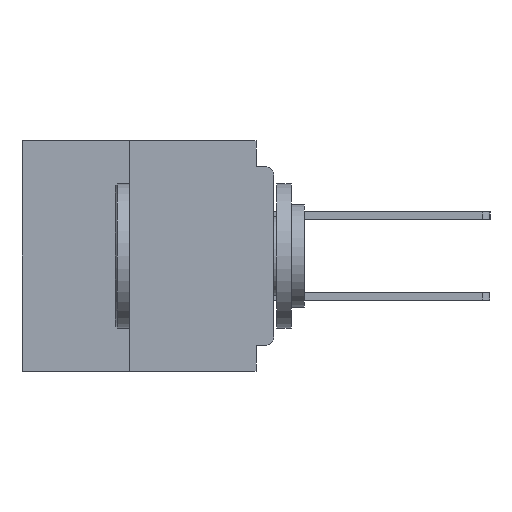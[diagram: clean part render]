
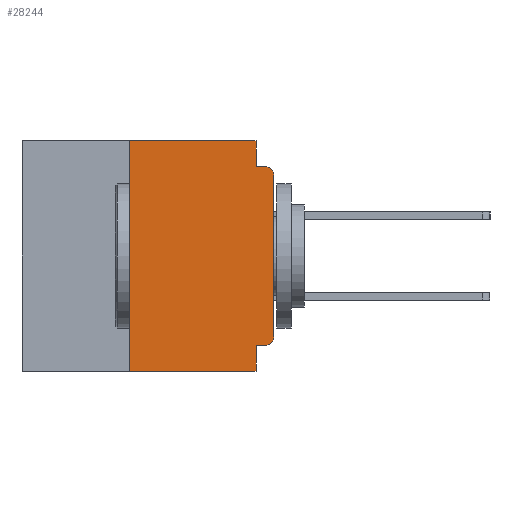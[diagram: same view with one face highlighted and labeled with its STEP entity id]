
A CAD part, left-side view. The second image highlights one B-rep face of the part: STEP entity #28244.
In plain terms, the highlighted planar face has unit normal (-1, 0, 0).
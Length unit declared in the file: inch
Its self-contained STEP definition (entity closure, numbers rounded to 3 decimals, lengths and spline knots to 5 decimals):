
#3299 = VERTEX_POINT ( 'NONE', #6352 ) ;
#4492 = VERTEX_POINT ( 'NONE', #36273 ) ;
#4686 = LINE ( 'NONE', #56543, #41906 ) ;
#5958 = ORIENTED_EDGE ( 'NONE', *, *, #50875, .F. ) ;
#6352 = CARTESIAN_POINT ( 'NONE',  ( 0., 0.25, -0.4 ) ) ;
#6396 = VECTOR ( 'NONE', #30634, 39.37008 ) ;
#6397 = CARTESIAN_POINT ( 'NONE',  ( 0., 0.437, -0.4 ) ) ;
#6936 = VERTEX_POINT ( 'NONE', #59837 ) ;
#7879 = CARTESIAN_POINT ( 'NONE',  ( 0., 0.031, 0. ) ) ;
#8286 = CIRCLE ( 'NONE', #15188, 0.015 ) ;
#8714 = VECTOR ( 'NONE', #12414, 39.37008 ) ;
#9457 = VECTOR ( 'NONE', #51533, 39.37008 ) ;
#12106 = CARTESIAN_POINT ( 'NONE',  ( 0., 0.015, -0.06 ) ) ;
#12159 = CARTESIAN_POINT ( 'NONE',  ( 0., 0.031, -0.355 ) ) ;
#12284 = CARTESIAN_POINT ( 'NONE',  ( 0., 0., -0.06 ) ) ;
#12414 = DIRECTION ( 'NONE',  ( 0., 0., 1. ) ) ;
#13117 = CARTESIAN_POINT ( 'NONE',  ( 0., 0.437, 0. ) ) ;
#14204 = CARTESIAN_POINT ( 'NONE',  ( 0., 0.015, -0.34 ) ) ;
#14446 = LINE ( 'NONE', #50013, #53010 ) ;
#15188 = AXIS2_PLACEMENT_3D ( 'NONE', #12106, #45990, #17058 ) ;
#16441 = VERTEX_POINT ( 'NONE', #31870 ) ;
#16653 = VECTOR ( 'NONE', #46979, 39.37008 ) ;
#17058 = DIRECTION ( 'NONE',  ( 0., 0., -1. ) ) ;
#17889 = ORIENTED_EDGE ( 'NONE', *, *, #33131, .T. ) ;
#19119 = DIRECTION ( 'NONE',  ( 0., 0., -1. ) ) ;
#19390 = PLANE ( 'NONE',  #32075 ) ;
#22426 = LINE ( 'NONE', #7879, #9457 ) ;
#22611 = DIRECTION ( 'NONE',  ( 0., 1., 0. ) ) ;
#22678 = VERTEX_POINT ( 'NONE', #55974 ) ;
#22692 = VERTEX_POINT ( 'NONE', #27287 ) ;
#23366 = ORIENTED_EDGE ( 'NONE', *, *, #61705, .F. ) ;
#24251 = DIRECTION ( 'NONE',  ( 1., 0., 0. ) ) ;
#24573 = LINE ( 'NONE', #46707, #35919 ) ;
#24841 = LINE ( 'NONE', #54201, #49025 ) ;
#25578 = EDGE_CURVE ( 'NONE', #45578, #22692, #14446, .T. ) ;
#25692 = EDGE_CURVE ( 'NONE', #55652, #22692, #8286, .T. ) ;
#25916 = DIRECTION ( 'NONE',  ( 0., -1., 0. ) ) ;
#26908 = VERTEX_POINT ( 'NONE', #12159 ) ;
#27287 = CARTESIAN_POINT ( 'NONE',  ( 0., 0.015, -0.045 ) ) ;
#28244 = ADVANCED_FACE ( 'NONE', ( #46644 ), #19390, .F. ) ;
#29496 = LINE ( 'NONE', #13117, #16653 ) ;
#30634 = DIRECTION ( 'NONE',  ( 0., -1., 0. ) ) ;
#30737 = LINE ( 'NONE', #6397, #6396 ) ;
#31812 = ORIENTED_EDGE ( 'NONE', *, *, #25692, .T. ) ;
#31870 = CARTESIAN_POINT ( 'NONE',  ( 0., 0.015, -0.355 ) ) ;
#32075 = AXIS2_PLACEMENT_3D ( 'NONE', #48321, #24251, #57952 ) ;
#32225 = EDGE_CURVE ( 'NONE', #4492, #45578, #22426, .T. ) ;
#32539 = DIRECTION ( 'NONE',  ( 0., 0., 1. ) ) ;
#33131 = EDGE_CURVE ( 'NONE', #16441, #6936, #56261, .T. ) ;
#34154 = ORIENTED_EDGE ( 'NONE', *, *, #54915, .F. ) ;
#34274 = EDGE_CURVE ( 'NONE', #6936, #55652, #4686, .T. ) ;
#35284 = ORIENTED_EDGE ( 'NONE', *, *, #34274, .T. ) ;
#35889 = EDGE_LOOP ( 'NONE', ( #35284, #31812, #54810, #36004, #49642, #23366, #38032, #34154, #5958, #17889 ) ) ;
#35919 = VECTOR ( 'NONE', #22611, 39.37008 ) ;
#36004 = ORIENTED_EDGE ( 'NONE', *, *, #32225, .F. ) ;
#36273 = CARTESIAN_POINT ( 'NONE',  ( 0., 0.031, 0. ) ) ;
#38017 = CARTESIAN_POINT ( 'NONE',  ( 0., 0.031, -0.045 ) ) ;
#38032 = ORIENTED_EDGE ( 'NONE', *, *, #61901, .T. ) ;
#41906 = VECTOR ( 'NONE', #32539, 39.37008 ) ;
#45578 = VERTEX_POINT ( 'NONE', #38017 ) ;
#45990 = DIRECTION ( 'NONE',  ( -1., 0., 0. ) ) ;
#46644 = FACE_OUTER_BOUND ( 'NONE', #35889, .T. ) ;
#46707 = CARTESIAN_POINT ( 'NONE',  ( 0., 0., -0.355 ) ) ;
#46979 = DIRECTION ( 'NONE',  ( 0., -1., 0. ) ) ;
#48061 = DIRECTION ( 'NONE',  ( -1., 0., 0. ) ) ;
#48321 = CARTESIAN_POINT ( 'NONE',  ( 0., 0.437, 0. ) ) ;
#49025 = VECTOR ( 'NONE', #59006, 39.37008 ) ;
#49642 = ORIENTED_EDGE ( 'NONE', *, *, #53869, .F. ) ;
#50013 = CARTESIAN_POINT ( 'NONE',  ( 0., 0., -0.045 ) ) ;
#50875 = EDGE_CURVE ( 'NONE', #16441, #26908, #24573, .T. ) ;
#51533 = DIRECTION ( 'NONE',  ( 0., 0., -1. ) ) ;
#51940 = CARTESIAN_POINT ( 'NONE',  ( 0., 0.25, 0. ) ) ;
#53010 = VECTOR ( 'NONE', #25916, 39.37008 ) ;
#53869 = EDGE_CURVE ( 'NONE', #57840, #4492, #29496, .T. ) ;
#54201 = CARTESIAN_POINT ( 'NONE',  ( 0., 0.031, -0.4 ) ) ;
#54810 = ORIENTED_EDGE ( 'NONE', *, *, #25578, .F. ) ;
#54915 = EDGE_CURVE ( 'NONE', #26908, #22678, #24841, .T. ) ;
#55652 = VERTEX_POINT ( 'NONE', #12284 ) ;
#55668 = LINE ( 'NONE', #55957, #8714 ) ;
#55957 = CARTESIAN_POINT ( 'NONE',  ( 0., 0.25, -0.4 ) ) ;
#55974 = CARTESIAN_POINT ( 'NONE',  ( 0., 0.031, -0.4 ) ) ;
#56067 = AXIS2_PLACEMENT_3D ( 'NONE', #14204, #48061, #19119 ) ;
#56261 = CIRCLE ( 'NONE', #56067, 0.015 ) ;
#56543 = CARTESIAN_POINT ( 'NONE',  ( 0., 0., 0. ) ) ;
#57840 = VERTEX_POINT ( 'NONE', #51940 ) ;
#57952 = DIRECTION ( 'NONE',  ( 0., 0., -1. ) ) ;
#59006 = DIRECTION ( 'NONE',  ( 0., 0., -1. ) ) ;
#59837 = CARTESIAN_POINT ( 'NONE',  ( 0., 0., -0.34 ) ) ;
#61705 = EDGE_CURVE ( 'NONE', #3299, #57840, #55668, .T. ) ;
#61901 = EDGE_CURVE ( 'NONE', #3299, #22678, #30737, .T. ) ;
